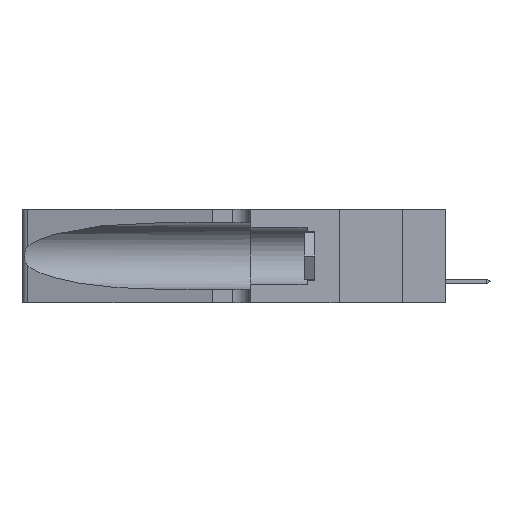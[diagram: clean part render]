
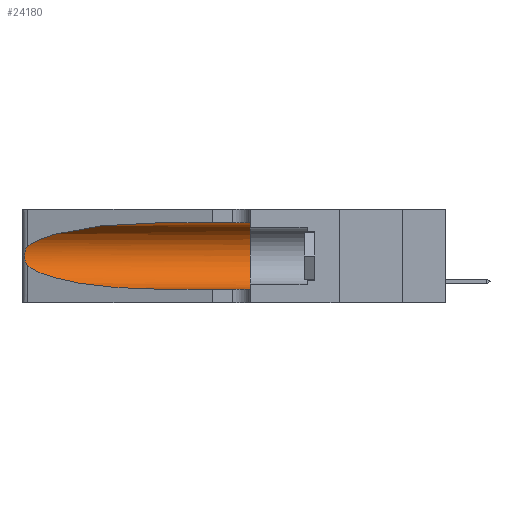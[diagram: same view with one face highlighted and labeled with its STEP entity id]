
A CAD part, left-side view. The second image highlights one B-rep face of the part: STEP entity #24180.
In plain terms, the highlighted cylindrical face has radius 3.308 mm (diameter 6.617 mm), a partial arc.
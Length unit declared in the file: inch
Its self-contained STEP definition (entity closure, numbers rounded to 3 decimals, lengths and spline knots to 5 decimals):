
#229 = CARTESIAN_POINT ( 'NONE',  ( 0.1305, 1.61858, 0.185 ) ) ;
#418 = EDGE_CURVE ( 'NONE', #26757, #20356, #20056, .T. ) ;
#751 = VERTEX_POINT ( 'NONE', #28060 ) ;
#1108 = VECTOR ( 'NONE', #14270, 39.37008 ) ;
#2118 = EDGE_CURVE ( 'NONE', #751, #17166, #6004, .T. ) ;
#2579 = VERTEX_POINT ( 'NONE', #18782 ) ;
#2881 = DIRECTION ( 'NONE',  ( 0., 0., -1. ) ) ;
#3160 = VECTOR ( 'NONE', #12959, 39.37008 ) ;
#3326 = CARTESIAN_POINT ( 'NONE',  ( 0.2373, 1.15595, 0.08982 ) ) ;
#4253 = CARTESIAN_POINT ( 'NONE',  ( 0.26075, 1.23896, 0.178 ) ) ;
#4303 = ORIENTED_EDGE ( 'NONE', *, *, #32575, .F. ) ;
#4344 = CYLINDRICAL_SURFACE ( 'NONE', #32240, 0.13025 ) ;
#5953 = CARTESIAN_POINT ( 'NONE',  ( 0.18966, 0.96281, 0.05475 ) ) ;
#6004 = LINE ( 'NONE', #18244, #3160 ) ;
#6284 = CARTESIAN_POINT ( 'NONE',  ( 0.1305, 0.72297, 0.31525 ) ) ;
#6516 = CARTESIAN_POINT ( 'NONE',  ( 0.25856, 1.23593, 0.16098 ) ) ;
#6618 = CARTESIAN_POINT ( 'NONE',  ( 0.25639, 1.23186, 0.15144 ) ) ;
#7602 = EDGE_LOOP ( 'NONE', ( #14018, #29347, #12077, #15910, #4303, #24165 ) ) ;
#7967 = VERTEX_POINT ( 'NONE', #17567 ) ;
#8932 = CARTESIAN_POINT ( 'NONE',  ( 0.25487, 1.22718, 0.22369 ) ) ;
#9037 = CARTESIAN_POINT ( 'NONE',  ( 0.25487, 1.22718, 0.22369 ) ) ;
#9149 = CARTESIAN_POINT ( 'NONE',  ( 0.25789, 1.23486, 0.15765 ) ) ;
#9770 = EDGE_CURVE ( 'NONE', #2579, #751, #17047, .T. ) ;
#11773 = CARTESIAN_POINT ( 'NONE',  ( 0.25487, 1.22718, 0.14631 ) ) ;
#12077 = ORIENTED_EDGE ( 'NONE', *, *, #9770, .T. ) ;
#12465 = CARTESIAN_POINT ( 'NONE',  ( 0.1305, 0.72297, 0.31525 ) ) ;
#12959 = DIRECTION ( 'NONE',  ( 0., -1., 0. ) ) ;
#13739 = FACE_OUTER_BOUND ( 'NONE', #7602, .T. ) ;
#13986 = CARTESIAN_POINT ( 'NONE',  ( 0.1305, 0.72297, 0.05475 ) ) ;
#14018 = ORIENTED_EDGE ( 'NONE', *, *, #14842, .T. ) ;
#14270 = DIRECTION ( 'NONE',  ( 0., -1., 0. ) ) ;
#14432 = CARTESIAN_POINT ( 'NONE',  ( 0.26017, 1.23833, 0.17102 ) ) ;
#14842 = EDGE_CURVE ( 'NONE', #26757, #7967, #15135, .T. ) ;
#15135 =( BOUNDED_CURVE ( )  B_SPLINE_CURVE ( 3, ( #6284, #17091, #24706, #8932 ),
 .UNSPECIFIED., .F., .F. ) 
 B_SPLINE_CURVE_WITH_KNOTS ( ( 4, 4 ),
 ( 1.5708, 2.84003 ),
 .UNSPECIFIED. ) 
 CURVE ( )  GEOMETRIC_REPRESENTATION_ITEM ( )  RATIONAL_B_SPLINE_CURVE ( ( 1., 0.87, 0.87, 1. ) ) 
 REPRESENTATION_ITEM ( '' )  );
#15910 = ORIENTED_EDGE ( 'NONE', *, *, #2118, .T. ) ;
#17047 =( BOUNDED_CURVE ( )  B_SPLINE_CURVE ( 3, ( #29849, #3326, #5953, #13986 ),
 .UNSPECIFIED., .F., .F. ) 
 B_SPLINE_CURVE_WITH_KNOTS ( ( 4, 4 ),
 ( 3.44316, 4.71239 ),
 .UNSPECIFIED. ) 
 CURVE ( )  GEOMETRIC_REPRESENTATION_ITEM ( )  RATIONAL_B_SPLINE_CURVE ( ( 1., 0.87, 0.87, 1. ) ) 
 REPRESENTATION_ITEM ( '' )  );
#17091 = CARTESIAN_POINT ( 'NONE',  ( 0.18966, 0.96281, 0.31525 ) ) ;
#17166 = VERTEX_POINT ( 'NONE', #18828 ) ;
#17202 = CARTESIAN_POINT ( 'NONE',  ( 0.25639, 1.23184, 0.21858 ) ) ;
#17567 = CARTESIAN_POINT ( 'NONE',  ( 0.25487, 1.22718, 0.22369 ) ) ;
#18066 = CIRCLE ( 'NONE', #32201, 0.13025 ) ;
#18244 = CARTESIAN_POINT ( 'NONE',  ( 0.1305, 1.61858, 0.05475 ) ) ;
#18611 = DIRECTION ( 'NONE',  ( 0., -1., 0. ) ) ;
#18782 = CARTESIAN_POINT ( 'NONE',  ( 0.25487, 1.22718, 0.14631 ) ) ;
#18828 = CARTESIAN_POINT ( 'NONE',  ( 0.1305, 0.35, 0.05475 ) ) ;
#19489 = DIRECTION ( 'NONE',  ( 0., 1., 0. ) ) ;
#19645 = CARTESIAN_POINT ( 'NONE',  ( 0.25555, 1.22994, 0.2215 ) ) ;
#19876 = CARTESIAN_POINT ( 'NONE',  ( 0.25787, 1.23484, 0.2124 ) ) ;
#20056 = LINE ( 'NONE', #32556, #1108 ) ;
#20356 = VERTEX_POINT ( 'NONE', #31121 ) ;
#22187 = CARTESIAN_POINT ( 'NONE',  ( 0.25555, 1.22993, 0.14849 ) ) ;
#22291 = CARTESIAN_POINT ( 'NONE',  ( 0.25854, 1.2359, 0.20912 ) ) ;
#24165 = ORIENTED_EDGE ( 'NONE', *, *, #418, .F. ) ;
#24180 = ADVANCED_FACE ( 'NONE', ( #13739 ), #4344, .F. ) ;
#24239 = B_SPLINE_CURVE_WITH_KNOTS ( 'NONE', 3,
 ( #9037, #19645, #17202, #19876, #22291, #25283, #30087, #4253, #14432, #6516, #9149, #6618, #22187, #11773 ),
 .UNSPECIFIED., .F., .F.,
 ( 4, 2, 2, 2, 2, 2, 4 ),
 ( 0., 0.00027, 0.00053, 0.00107, 0.0016, 0.00187, 0.00214 ),
 .UNSPECIFIED. ) ;
#24565 = CARTESIAN_POINT ( 'NONE',  ( 0.1305, 0.35, 0.185 ) ) ;
#24706 = CARTESIAN_POINT ( 'NONE',  ( 0.2373, 1.15595, 0.28018 ) ) ;
#25283 = CARTESIAN_POINT ( 'NONE',  ( 0.26018, 1.23835, 0.19895 ) ) ;
#26757 = VERTEX_POINT ( 'NONE', #12465 ) ;
#27159 = DIRECTION ( 'NONE',  ( 0., 0., 1. ) ) ;
#28060 = CARTESIAN_POINT ( 'NONE',  ( 0.1305, 0.72297, 0.05475 ) ) ;
#29347 = ORIENTED_EDGE ( 'NONE', *, *, #31987, .T. ) ;
#29849 = CARTESIAN_POINT ( 'NONE',  ( 0.25487, 1.22718, 0.14631 ) ) ;
#30087 = CARTESIAN_POINT ( 'NONE',  ( 0.26075, 1.23896, 0.19203 ) ) ;
#31121 = CARTESIAN_POINT ( 'NONE',  ( 0.1305, 0.35, 0.31525 ) ) ;
#31987 = EDGE_CURVE ( 'NONE', #7967, #2579, #24239, .T. ) ;
#32201 = AXIS2_PLACEMENT_3D ( 'NONE', #24565, #19489, #27159 ) ;
#32240 = AXIS2_PLACEMENT_3D ( 'NONE', #229, #18611, #2881 ) ;
#32556 = CARTESIAN_POINT ( 'NONE',  ( 0.1305, 1.61858, 0.31525 ) ) ;
#32575 = EDGE_CURVE ( 'NONE', #20356, #17166, #18066, .T. ) ;
